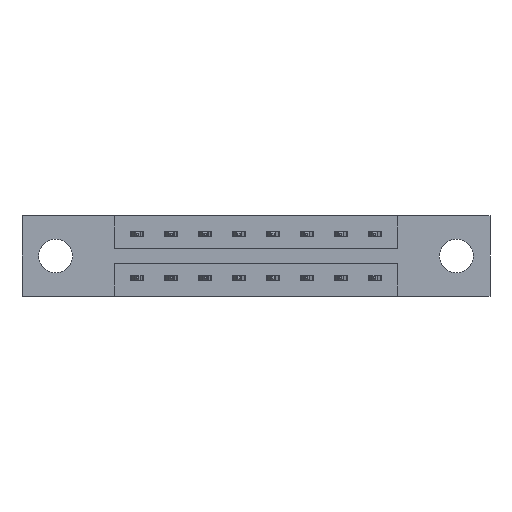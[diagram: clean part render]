
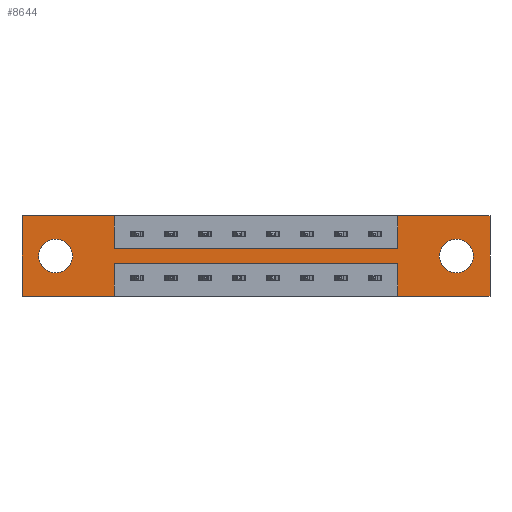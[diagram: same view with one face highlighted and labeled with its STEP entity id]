
A CAD part, front view. The second image highlights one B-rep face of the part: STEP entity #8644.
In plain terms, the highlighted planar face has unit normal (0, -1, 0).
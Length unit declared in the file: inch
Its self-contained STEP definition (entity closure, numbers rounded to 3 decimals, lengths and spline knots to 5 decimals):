
#19 = ORIENTED_EDGE ( 'NONE', *, *, #106, .F. ) ;
#31 = LINE ( 'NONE', #4105, #6755 ) ;
#37 = VECTOR ( 'NONE', #6325, 39.37008 ) ;
#86 = AXIS2_PLACEMENT_3D ( 'NONE', #9779, #8256, #9929 ) ;
#106 = EDGE_CURVE ( 'NONE', #9471, #2361, #10037, .T. ) ;
#146 = VERTEX_POINT ( 'NONE', #5989 ) ;
#181 = EDGE_CURVE ( 'NONE', #8970, #4938, #31, .T. ) ;
#417 = CARTESIAN_POINT ( 'NONE',  ( 0.155, 0., -0.107 ) ) ;
#432 = DIRECTION ( 'NONE',  ( 1., 0., 0. ) ) ;
#467 = ORIENTED_EDGE ( 'NONE', *, *, #7324, .F. ) ;
#486 = DIRECTION ( 'NONE',  ( 0., 1., 0. ) ) ;
#533 = DIRECTION ( 'NONE',  ( -1., 0., 0. ) ) ;
#539 = LINE ( 'NONE', #7178, #9522 ) ;
#611 = VECTOR ( 'NONE', #9112, 39.37008 ) ;
#663 = CARTESIAN_POINT ( 'NONE',  ( 0.425, 0., -0.22 ) ) ;
#666 = AXIS2_PLACEMENT_3D ( 'NONE', #6986, #486, #7806 ) ;
#791 = CARTESIAN_POINT ( 'NONE',  ( 0.425, 0., -0.37 ) ) ;
#819 = DIRECTION ( 'NONE',  ( 0., 1., 0. ) ) ;
#887 = CIRCLE ( 'NONE', #666, 0.078 ) ;
#1152 = CARTESIAN_POINT ( 'NONE',  ( 1.999, 0., -0.107 ) ) ;
#1156 = LINE ( 'NONE', #663, #37 ) ;
#1158 = CARTESIAN_POINT ( 'NONE',  ( 0., 0., 0. ) ) ;
#1288 = EDGE_CURVE ( 'NONE', #2361, #6244, #7003, .T. ) ;
#1555 = CARTESIAN_POINT ( 'NONE',  ( 1.729, 0., -0.37 ) ) ;
#1560 = DIRECTION ( 'NONE',  ( -1., 0., 0. ) ) ;
#1654 = DIRECTION ( 'NONE',  ( 0., 0., -1. ) ) ;
#1718 = CARTESIAN_POINT ( 'NONE',  ( 1.729, 0., 0. ) ) ;
#1813 = CARTESIAN_POINT ( 'NONE',  ( 1.999, 0., -0.185 ) ) ;
#1924 = CARTESIAN_POINT ( 'NONE',  ( 0.425, 0., -0.22 ) ) ;
#1994 = ORIENTED_EDGE ( 'NONE', *, *, #9717, .F. ) ;
#2057 = CIRCLE ( 'NONE', #9591, 0.078 ) ;
#2128 = EDGE_LOOP ( 'NONE', ( #7971, #8588, #6646, #467, #10146, #3135, #19, #1994, #5692, #3000, #10576, #7967 ) ) ;
#2321 = EDGE_CURVE ( 'NONE', #5150, #3491, #2769, .T. ) ;
#2343 = CIRCLE ( 'NONE', #6654, 0.078 ) ;
#2361 = VERTEX_POINT ( 'NONE', #7238 ) ;
#2533 = DIRECTION ( 'NONE',  ( 0., 0., -1. ) ) ;
#2673 = VECTOR ( 'NONE', #6516, 39.37008 ) ;
#2675 = ORIENTED_EDGE ( 'NONE', *, *, #2321, .T. ) ;
#2727 = DIRECTION ( 'NONE',  ( 0., 0., 1. ) ) ;
#2752 = DIRECTION ( 'NONE',  ( 0., 1., 0. ) ) ;
#2767 = VECTOR ( 'NONE', #6875, 39.37008 ) ;
#2769 = CIRCLE ( 'NONE', #6647, 0.078 ) ;
#3000 = ORIENTED_EDGE ( 'NONE', *, *, #7263, .F. ) ;
#3018 = FACE_BOUND ( 'NONE', #5132, .T. ) ;
#3035 = EDGE_CURVE ( 'NONE', #3491, #5150, #2343, .T. ) ;
#3135 = ORIENTED_EDGE ( 'NONE', *, *, #1288, .F. ) ;
#3211 = CARTESIAN_POINT ( 'NONE',  ( 0.425, 0., 0. ) ) ;
#3323 = DIRECTION ( 'NONE',  ( 0., 0., 1. ) ) ;
#3450 = CARTESIAN_POINT ( 'NONE',  ( 0., 0., -0.37 ) ) ;
#3491 = VERTEX_POINT ( 'NONE', #1152 ) ;
#3569 = VERTEX_POINT ( 'NONE', #1924 ) ;
#3833 = CARTESIAN_POINT ( 'NONE',  ( 2.154, 0., -0.37 ) ) ;
#4009 = PLANE ( 'NONE',  #86 ) ;
#4048 = EDGE_CURVE ( 'NONE', #146, #8166, #2057, .T. ) ;
#4049 = CARTESIAN_POINT ( 'NONE',  ( 0., 0., -0.37 ) ) ;
#4105 = CARTESIAN_POINT ( 'NONE',  ( 0.425, 0., 0. ) ) ;
#4144 = CARTESIAN_POINT ( 'NONE',  ( 0., 0., 0. ) ) ;
#4195 = CARTESIAN_POINT ( 'NONE',  ( 1.729, 0., -0.37 ) ) ;
#4386 = DIRECTION ( 'NONE',  ( 0., 0., -1. ) ) ;
#4432 = CARTESIAN_POINT ( 'NONE',  ( 0.425, 0., -0.15 ) ) ;
#4781 = EDGE_CURVE ( 'NONE', #6244, #7284, #539, .T. ) ;
#4824 = EDGE_CURVE ( 'NONE', #6345, #3569, #1156, .T. ) ;
#4879 = CARTESIAN_POINT ( 'NONE',  ( 1.729, 0., -0.15 ) ) ;
#4938 = VERTEX_POINT ( 'NONE', #5732 ) ;
#5039 = VERTEX_POINT ( 'NONE', #4195 ) ;
#5132 = EDGE_LOOP ( 'NONE', ( #7195, #8104 ) ) ;
#5150 = VERTEX_POINT ( 'NONE', #6159 ) ;
#5190 = LINE ( 'NONE', #8745, #6460 ) ;
#5307 = LINE ( 'NONE', #1158, #10510 ) ;
#5654 = CARTESIAN_POINT ( 'NONE',  ( 0.425, 0., -0.37 ) ) ;
#5692 = ORIENTED_EDGE ( 'NONE', *, *, #181, .F. ) ;
#5732 = CARTESIAN_POINT ( 'NONE',  ( 0.425, 0., -0.15 ) ) ;
#5793 = VERTEX_POINT ( 'NONE', #3450 ) ;
#5921 = FACE_OUTER_BOUND ( 'NONE', #2128, .T. ) ;
#5930 = CARTESIAN_POINT ( 'NONE',  ( 1.729, 0., -0.22 ) ) ;
#5989 = CARTESIAN_POINT ( 'NONE',  ( 0.155, 0., -0.263 ) ) ;
#6010 = EDGE_CURVE ( 'NONE', #8166, #146, #887, .T. ) ;
#6048 = FACE_BOUND ( 'NONE', #8509, .T. ) ;
#6159 = CARTESIAN_POINT ( 'NONE',  ( 1.999, 0., -0.263 ) ) ;
#6192 = LINE ( 'NONE', #4144, #611 ) ;
#6217 = EDGE_CURVE ( 'NONE', #9881, #5793, #6731, .T. ) ;
#6244 = VERTEX_POINT ( 'NONE', #6509 ) ;
#6325 = DIRECTION ( 'NONE',  ( -1., 0., 0. ) ) ;
#6345 = VERTEX_POINT ( 'NONE', #5930 ) ;
#6460 = VECTOR ( 'NONE', #533, 39.37008 ) ;
#6488 = VECTOR ( 'NONE', #1560, 39.37008 ) ;
#6509 = CARTESIAN_POINT ( 'NONE',  ( 2.154, 0., 0. ) ) ;
#6516 = DIRECTION ( 'NONE',  ( 1., 0., 0. ) ) ;
#6575 = DIRECTION ( 'NONE',  ( 0., 0., -1. ) ) ;
#6583 = LINE ( 'NONE', #4432, #2767 ) ;
#6646 = ORIENTED_EDGE ( 'NONE', *, *, #8963, .F. ) ;
#6647 = AXIS2_PLACEMENT_3D ( 'NONE', #9857, #819, #1654 ) ;
#6654 = AXIS2_PLACEMENT_3D ( 'NONE', #1813, #2752, #4386 ) ;
#6656 = VERTEX_POINT ( 'NONE', #10478 ) ;
#6731 = LINE ( 'NONE', #4049, #6488 ) ;
#6755 = VECTOR ( 'NONE', #6575, 39.37008 ) ;
#6875 = DIRECTION ( 'NONE',  ( 1., 0., 0. ) ) ;
#6986 = CARTESIAN_POINT ( 'NONE',  ( 0.155, 0., -0.185 ) ) ;
#7003 = LINE ( 'NONE', #9008, #2673 ) ;
#7178 = CARTESIAN_POINT ( 'NONE',  ( 2.154, 0., 0. ) ) ;
#7195 = ORIENTED_EDGE ( 'NONE', *, *, #6010, .T. ) ;
#7238 = CARTESIAN_POINT ( 'NONE',  ( 1.729, 0., 0. ) ) ;
#7263 = EDGE_CURVE ( 'NONE', #6656, #8970, #5307, .T. ) ;
#7284 = VERTEX_POINT ( 'NONE', #3833 ) ;
#7324 = EDGE_CURVE ( 'NONE', #7284, #5039, #5190, .T. ) ;
#7800 = VECTOR ( 'NONE', #2727, 39.37008 ) ;
#7806 = DIRECTION ( 'NONE',  ( 0., 0., 1. ) ) ;
#7967 = ORIENTED_EDGE ( 'NONE', *, *, #6217, .F. ) ;
#7971 = ORIENTED_EDGE ( 'NONE', *, *, #9930, .F. ) ;
#8022 = DIRECTION ( 'NONE',  ( 0., 0., -1. ) ) ;
#8104 = ORIENTED_EDGE ( 'NONE', *, *, #4048, .T. ) ;
#8166 = VERTEX_POINT ( 'NONE', #417 ) ;
#8182 = DIRECTION ( 'NONE',  ( 0., 0., 1. ) ) ;
#8256 = DIRECTION ( 'NONE',  ( 0., -1., 0. ) ) ;
#8294 = LINE ( 'NONE', #1555, #9337 ) ;
#8509 = EDGE_LOOP ( 'NONE', ( #9892, #2675 ) ) ;
#8588 = ORIENTED_EDGE ( 'NONE', *, *, #4824, .F. ) ;
#8644 = ADVANCED_FACE ( 'NONE', ( #6048, #3018, #5921 ), #4009, .T. ) ;
#8745 = CARTESIAN_POINT ( 'NONE',  ( 0., 0., -0.37 ) ) ;
#8942 = VECTOR ( 'NONE', #2533, 39.37008 ) ;
#8963 = EDGE_CURVE ( 'NONE', #5039, #6345, #8294, .T. ) ;
#8970 = VERTEX_POINT ( 'NONE', #3211 ) ;
#9008 = CARTESIAN_POINT ( 'NONE',  ( 0., 0., 0. ) ) ;
#9018 = EDGE_CURVE ( 'NONE', #5793, #6656, #6192, .T. ) ;
#9038 = DIRECTION ( 'NONE',  ( 0., 1., 0. ) ) ;
#9112 = DIRECTION ( 'NONE',  ( 0., 0., 1. ) ) ;
#9337 = VECTOR ( 'NONE', #8182, 39.37008 ) ;
#9463 = LINE ( 'NONE', #791, #8942 ) ;
#9471 = VERTEX_POINT ( 'NONE', #4879 ) ;
#9522 = VECTOR ( 'NONE', #8022, 39.37008 ) ;
#9591 = AXIS2_PLACEMENT_3D ( 'NONE', #9818, #9038, #3323 ) ;
#9717 = EDGE_CURVE ( 'NONE', #4938, #9471, #6583, .T. ) ;
#9779 = CARTESIAN_POINT ( 'NONE',  ( 0., 0., -0.37 ) ) ;
#9818 = CARTESIAN_POINT ( 'NONE',  ( 0.155, 0., -0.185 ) ) ;
#9857 = CARTESIAN_POINT ( 'NONE',  ( 1.999, 0., -0.185 ) ) ;
#9881 = VERTEX_POINT ( 'NONE', #5654 ) ;
#9892 = ORIENTED_EDGE ( 'NONE', *, *, #3035, .T. ) ;
#9929 = DIRECTION ( 'NONE',  ( 0., 0., -1. ) ) ;
#9930 = EDGE_CURVE ( 'NONE', #3569, #9881, #9463, .T. ) ;
#10037 = LINE ( 'NONE', #1718, #7800 ) ;
#10146 = ORIENTED_EDGE ( 'NONE', *, *, #4781, .F. ) ;
#10478 = CARTESIAN_POINT ( 'NONE',  ( 0., 0., 0. ) ) ;
#10510 = VECTOR ( 'NONE', #432, 39.37008 ) ;
#10576 = ORIENTED_EDGE ( 'NONE', *, *, #9018, .F. ) ;
